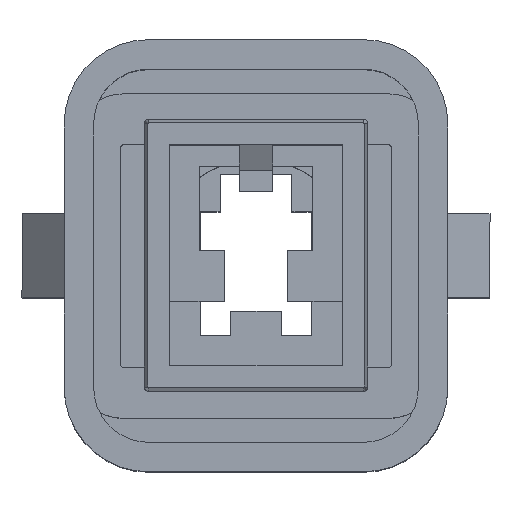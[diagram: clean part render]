
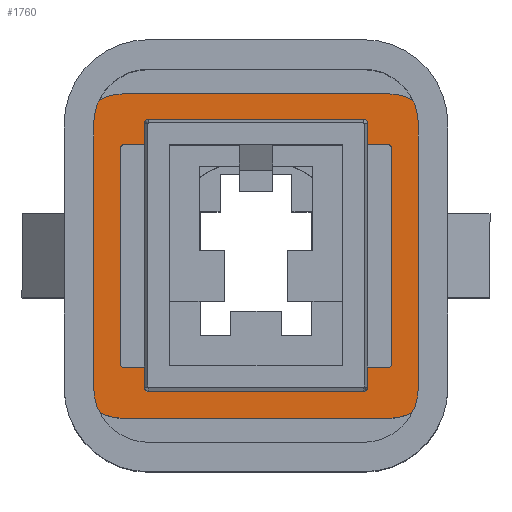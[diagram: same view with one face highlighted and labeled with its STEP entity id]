
A CAD part, top view. The second image highlights one B-rep face of the part: STEP entity #1760.
In plain terms, the highlighted planar face has unit normal (0, 0, 1).
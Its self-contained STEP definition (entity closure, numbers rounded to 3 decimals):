
#11 = EDGE_CURVE ( 'NONE', #5127, #5507, #512, .T. ) ;
#55 = CIRCLE ( 'NONE', #4404, 0.1 ) ;
#184 = CARTESIAN_POINT ( 'NONE',  ( 3.125, 3.85, -0.265 ) ) ;
#273 = CARTESIAN_POINT ( 'NONE',  ( 3.125, -3.85, -0.265 ) ) ;
#375 = CARTESIAN_POINT ( 'NONE',  ( -3.125, -2.55, -0.265 ) ) ;
#382 = EDGE_CURVE ( 'NONE', #3778, #1416, #1659, .T. ) ;
#402 = DIRECTION ( 'NONE',  ( -1., 0., 0. ) ) ;
#414 = AXIS2_PLACEMENT_3D ( 'NONE', #1336, #2129, #4801 ) ;
#427 = CARTESIAN_POINT ( 'NONE',  ( -3.125, -2.65, -0.265 ) ) ;
#456 = ORIENTED_EDGE ( 'NONE', *, *, #3463, .T. ) ;
#461 = CARTESIAN_POINT ( 'NONE',  ( 3.125, -3.85, -0.265 ) ) ;
#470 = FACE_OUTER_BOUND ( 'NONE', #1253, .T. ) ;
#492 = CARTESIAN_POINT ( 'NONE',  ( 4.425, 2.55, -0.265 ) ) ;
#512 = LINE ( 'NONE', #3575, #5071 ) ;
#594 = ORIENTED_EDGE ( 'NONE', *, *, #2771, .T. ) ;
#635 = CARTESIAN_POINT ( 'NONE',  ( 3.125, -2.65, -0.265 ) ) ;
#676 = CARTESIAN_POINT ( 'NONE',  ( -3.125, 2.55, -0.265 ) ) ;
#678 = EDGE_LOOP ( 'NONE', ( #2944, #3458, #1062, #456, #5141, #4457, #2363, #1133 ) ) ;
#695 = DIRECTION ( 'NONE',  ( 0., 1., 0. ) ) ;
#719 = AXIS2_PLACEMENT_3D ( 'NONE', #1678, #924, #4266 ) ;
#776 = DIRECTION ( 'NONE',  ( -1., 0., 0. ) ) ;
#789 = DIRECTION ( 'NONE',  ( -1., 0., 0. ) ) ;
#827 = ORIENTED_EDGE ( 'NONE', *, *, #3977, .F. ) ;
#878 = CARTESIAN_POINT ( 'NONE',  ( -3.225, -2.55, -0.265 ) ) ;
#901 = VECTOR ( 'NONE', #2430, 1000. ) ;
#924 = DIRECTION ( 'NONE',  ( 0., 0., -1. ) ) ;
#1061 = LINE ( 'NONE', #1428, #3336 ) ;
#1062 = ORIENTED_EDGE ( 'NONE', *, *, #3181, .T. ) ;
#1101 = ORIENTED_EDGE ( 'NONE', *, *, #3483, .F. ) ;
#1133 = ORIENTED_EDGE ( 'NONE', *, *, #2408, .T. ) ;
#1180 = DIRECTION ( 'NONE',  ( 0., 0., -1. ) ) ;
#1183 = EDGE_CURVE ( 'NONE', #5507, #5248, #3606, .T. ) ;
#1194 = CARTESIAN_POINT ( 'NONE',  ( 3.125, 2.65, -0.265 ) ) ;
#1253 = EDGE_LOOP ( 'NONE', ( #594, #4746, #4403, #827, #3245, #3315, #1862, #1101 ) ) ;
#1267 = VERTEX_POINT ( 'NONE', #4036 ) ;
#1284 = PLANE ( 'NONE',  #719 ) ;
#1325 = CARTESIAN_POINT ( 'NONE',  ( 4.425, -2.55, -0.265 ) ) ;
#1336 = CARTESIAN_POINT ( 'NONE',  ( 3.125, -2.55, -0.265 ) ) ;
#1416 = VERTEX_POINT ( 'NONE', #3294 ) ;
#1428 = CARTESIAN_POINT ( 'NONE',  ( -4.425, -2.55, -0.265 ) ) ;
#1456 = VERTEX_POINT ( 'NONE', #1532 ) ;
#1498 = DIRECTION ( 'NONE',  ( -1., 0., 0. ) ) ;
#1521 = CIRCLE ( 'NONE', #3801, 0.1 ) ;
#1532 = CARTESIAN_POINT ( 'NONE',  ( 3.125, 3.85, -0.265 ) ) ;
#1536 = CARTESIAN_POINT ( 'NONE',  ( -4.425, 2.55, -0.265 ) ) ;
#1659 = LINE ( 'NONE', #2560, #2194 ) ;
#1678 = CARTESIAN_POINT ( 'NONE',  ( 3.125, 2.65, -0.265 ) ) ;
#1703 = EDGE_CURVE ( 'NONE', #2027, #1267, #2850, .T. ) ;
#1760 = ADVANCED_FACE ( 'NONE', ( #4714, #470 ), #1284, .F. ) ;
#1846 = LINE ( 'NONE', #635, #3340 ) ;
#1862 = ORIENTED_EDGE ( 'NONE', *, *, #11, .F. ) ;
#1900 = CARTESIAN_POINT ( 'NONE',  ( 3.225, -2.55, -0.265 ) ) ;
#1910 = DIRECTION ( 'NONE',  ( -1., 0., 0. ) ) ;
#1969 = VECTOR ( 'NONE', #789, 1000. ) ;
#2027 = VERTEX_POINT ( 'NONE', #1536 ) ;
#2055 = DIRECTION ( 'NONE',  ( -1., 0., 0. ) ) ;
#2057 = CIRCLE ( 'NONE', #5238, 1.3 ) ;
#2070 = CARTESIAN_POINT ( 'NONE',  ( -3.125, -3.85, -0.265 ) ) ;
#2129 = DIRECTION ( 'NONE',  ( 0., 0., -1. ) ) ;
#2194 = VECTOR ( 'NONE', #5565, 1000. ) ;
#2235 = DIRECTION ( 'NONE',  ( 0., 0., -1. ) ) ;
#2267 = DIRECTION ( 'NONE',  ( 0., -1., 0. ) ) ;
#2343 = CIRCLE ( 'NONE', #2349, 0.1 ) ;
#2349 = AXIS2_PLACEMENT_3D ( 'NONE', #4510, #4927, #5380 ) ;
#2350 = DIRECTION ( 'NONE',  ( 0., 0., -1. ) ) ;
#2363 = ORIENTED_EDGE ( 'NONE', *, *, #382, .T. ) ;
#2408 = EDGE_CURVE ( 'NONE', #1416, #3923, #55, .T. ) ;
#2430 = DIRECTION ( 'NONE',  ( 0., -1., 0. ) ) ;
#2524 = DIRECTION ( 'NONE',  ( 0., 0., -1. ) ) ;
#2529 = CARTESIAN_POINT ( 'NONE',  ( -3.125, 2.55, -0.265 ) ) ;
#2560 = CARTESIAN_POINT ( 'NONE',  ( -3.225, -2.55, -0.265 ) ) ;
#2635 = EDGE_CURVE ( 'NONE', #4283, #2027, #1061, .T. ) ;
#2717 = CARTESIAN_POINT ( 'NONE',  ( -3.125, 2.65, -0.265 ) ) ;
#2771 = EDGE_CURVE ( 'NONE', #1456, #1267, #4073, .T. ) ;
#2838 = VERTEX_POINT ( 'NONE', #5449 ) ;
#2850 = CIRCLE ( 'NONE', #4751, 1.3 ) ;
#2944 = ORIENTED_EDGE ( 'NONE', *, *, #4072, .F. ) ;
#2969 = CIRCLE ( 'NONE', #4956, 1.3 ) ;
#3105 = EDGE_CURVE ( 'NONE', #4834, #3384, #1846, .T. ) ;
#3162 = VECTOR ( 'NONE', #1910, 1000. ) ;
#3181 = EDGE_CURVE ( 'NONE', #5446, #5323, #5496, .T. ) ;
#3232 = CARTESIAN_POINT ( 'NONE',  ( -3.125, -2.55, -0.265 ) ) ;
#3245 = ORIENTED_EDGE ( 'NONE', *, *, #3632, .F. ) ;
#3294 = CARTESIAN_POINT ( 'NONE',  ( -3.225, 2.55, -0.265 ) ) ;
#3315 = ORIENTED_EDGE ( 'NONE', *, *, #1183, .F. ) ;
#3336 = VECTOR ( 'NONE', #695, 1000. ) ;
#3340 = VECTOR ( 'NONE', #4064, 1000. ) ;
#3342 = CARTESIAN_POINT ( 'NONE',  ( 3.125, 2.55, -0.265 ) ) ;
#3360 = DIRECTION ( 'NONE',  ( 0., 0., -1. ) ) ;
#3384 = VERTEX_POINT ( 'NONE', #427 ) ;
#3458 = ORIENTED_EDGE ( 'NONE', *, *, #3692, .T. ) ;
#3463 = EDGE_CURVE ( 'NONE', #5323, #4834, #2343, .T. ) ;
#3483 = EDGE_CURVE ( 'NONE', #1456, #5127, #2969, .T. ) ;
#3515 = CARTESIAN_POINT ( 'NONE',  ( 3.225, 2.55, -0.265 ) ) ;
#3551 = CARTESIAN_POINT ( 'NONE',  ( 3.125, 2.55, -0.265 ) ) ;
#3575 = CARTESIAN_POINT ( 'NONE',  ( 4.425, 2.55, -0.265 ) ) ;
#3606 = CIRCLE ( 'NONE', #414, 1.3 ) ;
#3632 = EDGE_CURVE ( 'NONE', #5248, #5069, #3768, .T. ) ;
#3692 = EDGE_CURVE ( 'NONE', #2838, #5446, #1521, .T. ) ;
#3768 = LINE ( 'NONE', #273, #1969 ) ;
#3778 = VERTEX_POINT ( 'NONE', #878 ) ;
#3801 = AXIS2_PLACEMENT_3D ( 'NONE', #3342, #1180, #2055 ) ;
#3836 = VECTOR ( 'NONE', #776, 1000. ) ;
#3923 = VERTEX_POINT ( 'NONE', #2717 ) ;
#3971 = DIRECTION ( 'NONE',  ( -1., 0., 0. ) ) ;
#3977 = EDGE_CURVE ( 'NONE', #5069, #4283, #2057, .T. ) ;
#3997 = EDGE_CURVE ( 'NONE', #3384, #3778, #4873, .T. ) ;
#4036 = CARTESIAN_POINT ( 'NONE',  ( -3.125, 3.85, -0.265 ) ) ;
#4064 = DIRECTION ( 'NONE',  ( -1., 0., 0. ) ) ;
#4072 = EDGE_CURVE ( 'NONE', #2838, #3923, #5083, .T. ) ;
#4073 = LINE ( 'NONE', #184, #3162 ) ;
#4266 = DIRECTION ( 'NONE',  ( -1., 0., 0. ) ) ;
#4283 = VERTEX_POINT ( 'NONE', #4697 ) ;
#4403 = ORIENTED_EDGE ( 'NONE', *, *, #2635, .F. ) ;
#4404 = AXIS2_PLACEMENT_3D ( 'NONE', #2529, #5560, #5485 ) ;
#4409 = CARTESIAN_POINT ( 'NONE',  ( 3.125, -2.65, -0.265 ) ) ;
#4457 = ORIENTED_EDGE ( 'NONE', *, *, #3997, .T. ) ;
#4510 = CARTESIAN_POINT ( 'NONE',  ( 3.125, -2.55, -0.265 ) ) ;
#4697 = CARTESIAN_POINT ( 'NONE',  ( -4.425, -2.55, -0.265 ) ) ;
#4714 = FACE_BOUND ( 'NONE', #678, .T. ) ;
#4746 = ORIENTED_EDGE ( 'NONE', *, *, #1703, .F. ) ;
#4751 = AXIS2_PLACEMENT_3D ( 'NONE', #676, #3360, #5086 ) ;
#4794 = AXIS2_PLACEMENT_3D ( 'NONE', #375, #2524, #402 ) ;
#4801 = DIRECTION ( 'NONE',  ( -1., 0., 0. ) ) ;
#4834 = VERTEX_POINT ( 'NONE', #4409 ) ;
#4873 = CIRCLE ( 'NONE', #4794, 0.1 ) ;
#4927 = DIRECTION ( 'NONE',  ( 0., 0., -1. ) ) ;
#4956 = AXIS2_PLACEMENT_3D ( 'NONE', #3551, #2350, #1498 ) ;
#5069 = VERTEX_POINT ( 'NONE', #2070 ) ;
#5071 = VECTOR ( 'NONE', #2267, 1000. ) ;
#5073 = CARTESIAN_POINT ( 'NONE',  ( 3.225, 2.55, -0.265 ) ) ;
#5083 = LINE ( 'NONE', #1194, #3836 ) ;
#5086 = DIRECTION ( 'NONE',  ( -1., 0., 0. ) ) ;
#5127 = VERTEX_POINT ( 'NONE', #492 ) ;
#5141 = ORIENTED_EDGE ( 'NONE', *, *, #3105, .T. ) ;
#5238 = AXIS2_PLACEMENT_3D ( 'NONE', #3232, #2235, #3971 ) ;
#5248 = VERTEX_POINT ( 'NONE', #461 ) ;
#5323 = VERTEX_POINT ( 'NONE', #1900 ) ;
#5380 = DIRECTION ( 'NONE',  ( -1., 0., 0. ) ) ;
#5446 = VERTEX_POINT ( 'NONE', #3515 ) ;
#5449 = CARTESIAN_POINT ( 'NONE',  ( 3.125, 2.65, -0.265 ) ) ;
#5485 = DIRECTION ( 'NONE',  ( -1., 0., 0. ) ) ;
#5496 = LINE ( 'NONE', #5073, #901 ) ;
#5507 = VERTEX_POINT ( 'NONE', #1325 ) ;
#5560 = DIRECTION ( 'NONE',  ( 0., 0., -1. ) ) ;
#5565 = DIRECTION ( 'NONE',  ( 0., 1., 0. ) ) ;
